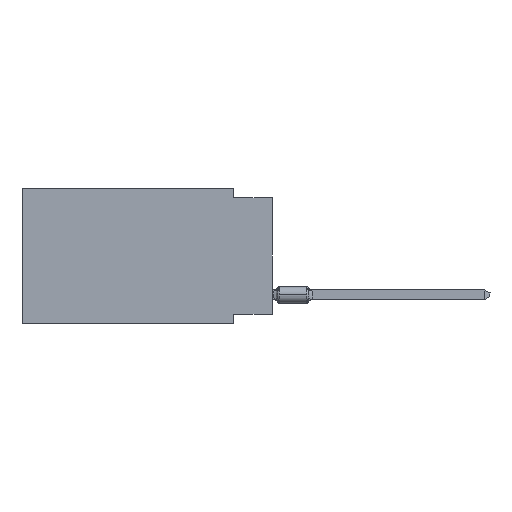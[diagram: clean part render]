
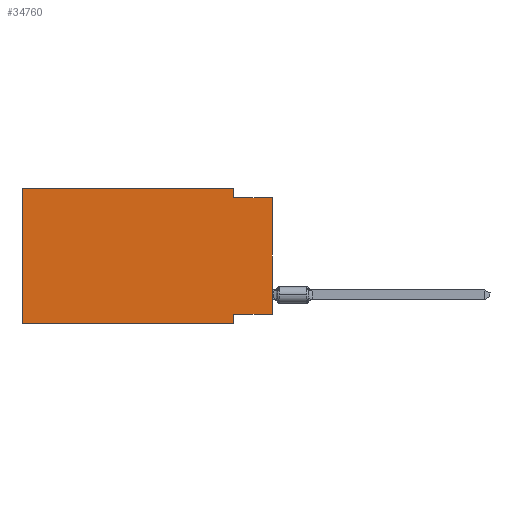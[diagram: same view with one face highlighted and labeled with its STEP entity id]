
A CAD part, left-side view. The second image highlights one B-rep face of the part: STEP entity #34760.
In plain terms, the highlighted planar face has unit normal (-1, 0, 0).
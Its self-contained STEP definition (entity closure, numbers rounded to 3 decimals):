
#601 = VECTOR ( 'NONE', #30020, 1000. ) ;
#612 = VERTEX_POINT ( 'NONE', #55577 ) ;
#820 = VECTOR ( 'NONE', #38089, 1000. ) ;
#860 = EDGE_CURVE ( 'NONE', #45325, #40290, #53678, .T. ) ;
#923 = VERTEX_POINT ( 'NONE', #51221 ) ;
#2033 = ORIENTED_EDGE ( 'NONE', *, *, #35677, .F. ) ;
#4031 = VECTOR ( 'NONE', #9777, 1000. ) ;
#4120 = VECTOR ( 'NONE', #13654, 1000. ) ;
#5831 = VERTEX_POINT ( 'NONE', #53632 ) ;
#6004 = LINE ( 'NONE', #34032, #35785 ) ;
#6767 = DIRECTION ( 'NONE',  ( 0., 1., 0. ) ) ;
#6850 = PLANE ( 'NONE',  #31190 ) ;
#7952 = DIRECTION ( 'NONE',  ( 0., 0., 1. ) ) ;
#8563 = VERTEX_POINT ( 'NONE', #38934 ) ;
#9167 = CARTESIAN_POINT ( 'NONE',  ( 0., 0., -0.635 ) ) ;
#9777 = DIRECTION ( 'NONE',  ( 0., 0., 1. ) ) ;
#10263 = EDGE_CURVE ( 'NONE', #51239, #8563, #12029, .T. ) ;
#10374 = LINE ( 'NONE', #51545, #4031 ) ;
#11331 = LINE ( 'NONE', #48531, #50265 ) ;
#12029 = LINE ( 'NONE', #25470, #601 ) ;
#13106 = EDGE_CURVE ( 'NONE', #612, #8563, #28342, .T. ) ;
#13654 = DIRECTION ( 'NONE',  ( 0., 0., -1. ) ) ;
#15098 = CARTESIAN_POINT ( 'NONE',  ( 0., 0., -8.255 ) ) ;
#15630 = EDGE_CURVE ( 'NONE', #30005, #923, #18541, .T. ) ;
#17056 = EDGE_LOOP ( 'NONE', ( #33956, #39901, #44314, #19062, #2033, #24564, #22106, #21883 ) ) ;
#18348 = VECTOR ( 'NONE', #42351, 1000. ) ;
#18541 = LINE ( 'NONE', #18832, #4120 ) ;
#18832 = CARTESIAN_POINT ( 'NONE',  ( 0., 2.54, 0. ) ) ;
#19062 = ORIENTED_EDGE ( 'NONE', *, *, #47579, .F. ) ;
#20869 = FACE_OUTER_BOUND ( 'NONE', #17056, .T. ) ;
#21883 = ORIENTED_EDGE ( 'NONE', *, *, #45970, .F. ) ;
#22106 = ORIENTED_EDGE ( 'NONE', *, *, #13106, .F. ) ;
#23776 = CARTESIAN_POINT ( 'NONE',  ( 0., 0., -0.635 ) ) ;
#24564 = ORIENTED_EDGE ( 'NONE', *, *, #10263, .T. ) ;
#24852 = CARTESIAN_POINT ( 'NONE',  ( 0., 16.383, 0. ) ) ;
#25470 = CARTESIAN_POINT ( 'NONE',  ( 0., 16.383, -8.89 ) ) ;
#28342 = LINE ( 'NONE', #56388, #820 ) ;
#30005 = VERTEX_POINT ( 'NONE', #54845 ) ;
#30020 = DIRECTION ( 'NONE',  ( 0., -1., 0. ) ) ;
#31190 = AXIS2_PLACEMENT_3D ( 'NONE', #24852, #38258, #57171 ) ;
#33956 = ORIENTED_EDGE ( 'NONE', *, *, #860, .T. ) ;
#34032 = CARTESIAN_POINT ( 'NONE',  ( 0., 16.383, 0. ) ) ;
#34760 = ADVANCED_FACE ( 'NONE', ( #20869 ), #6850, .F. ) ;
#35677 = EDGE_CURVE ( 'NONE', #51239, #5831, #10374, .T. ) ;
#35785 = VECTOR ( 'NONE', #57512, 1000. ) ;
#36277 = CARTESIAN_POINT ( 'NONE',  ( 0., 0., 0. ) ) ;
#38089 = DIRECTION ( 'NONE',  ( 0., 0., -1. ) ) ;
#38258 = DIRECTION ( 'NONE',  ( 1., 0., 0. ) ) ;
#38934 = CARTESIAN_POINT ( 'NONE',  ( 0., 2.54, -8.89 ) ) ;
#39901 = ORIENTED_EDGE ( 'NONE', *, *, #40982, .F. ) ;
#40290 = VERTEX_POINT ( 'NONE', #9167 ) ;
#40982 = EDGE_CURVE ( 'NONE', #923, #40290, #46947, .T. ) ;
#42351 = DIRECTION ( 'NONE',  ( 0., -1., 0. ) ) ;
#44314 = ORIENTED_EDGE ( 'NONE', *, *, #15630, .F. ) ;
#45325 = VERTEX_POINT ( 'NONE', #15098 ) ;
#45970 = EDGE_CURVE ( 'NONE', #45325, #612, #11331, .T. ) ;
#46947 = LINE ( 'NONE', #23776, #18348 ) ;
#47579 = EDGE_CURVE ( 'NONE', #5831, #30005, #6004, .T. ) ;
#48531 = CARTESIAN_POINT ( 'NONE',  ( 0., 0., -8.255 ) ) ;
#50265 = VECTOR ( 'NONE', #6767, 1000. ) ;
#50419 = VECTOR ( 'NONE', #7952, 1000. ) ;
#51221 = CARTESIAN_POINT ( 'NONE',  ( 0., 2.54, -0.635 ) ) ;
#51239 = VERTEX_POINT ( 'NONE', #53839 ) ;
#51545 = CARTESIAN_POINT ( 'NONE',  ( 0., 16.383, 0. ) ) ;
#53632 = CARTESIAN_POINT ( 'NONE',  ( 0., 16.383, 0. ) ) ;
#53678 = LINE ( 'NONE', #36277, #50419 ) ;
#53839 = CARTESIAN_POINT ( 'NONE',  ( 0., 16.383, -8.89 ) ) ;
#54845 = CARTESIAN_POINT ( 'NONE',  ( 0., 2.54, 0. ) ) ;
#55577 = CARTESIAN_POINT ( 'NONE',  ( 0., 2.54, -8.255 ) ) ;
#56388 = CARTESIAN_POINT ( 'NONE',  ( 0., 2.54, -8.89 ) ) ;
#57171 = DIRECTION ( 'NONE',  ( 0., 0., -1. ) ) ;
#57512 = DIRECTION ( 'NONE',  ( 0., -1., 0. ) ) ;
